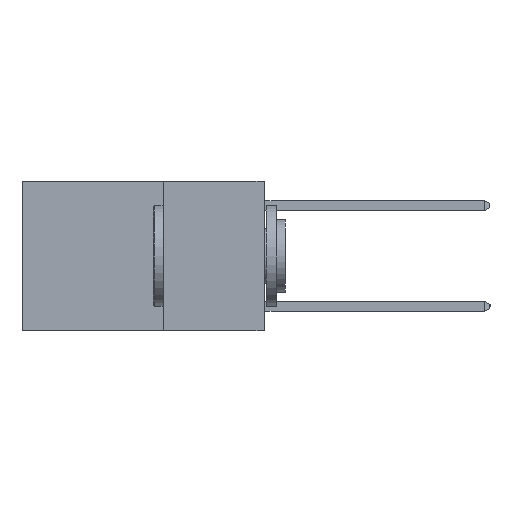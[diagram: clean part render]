
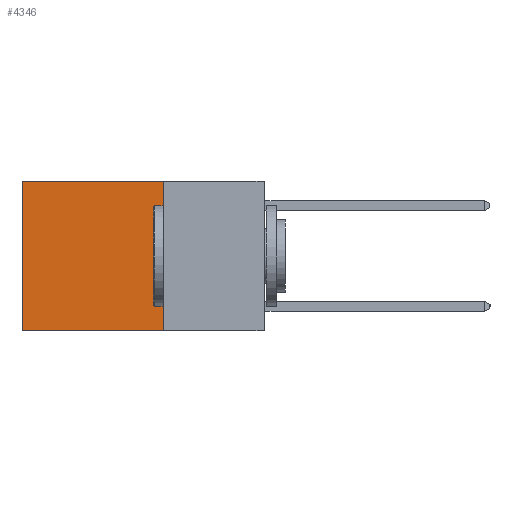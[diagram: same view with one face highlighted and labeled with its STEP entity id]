
A CAD part, left-side view. The second image highlights one B-rep face of the part: STEP entity #4346.
In plain terms, the highlighted planar face has unit normal (-1, 0, 0).
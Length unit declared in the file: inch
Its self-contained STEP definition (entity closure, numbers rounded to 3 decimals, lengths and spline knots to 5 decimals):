
#273 = LINE ( 'NONE', #6829, #2418 ) ;
#440 = EDGE_LOOP ( 'NONE', ( #10818, #9083, #8532, #10730 ) ) ;
#696 = CARTESIAN_POINT ( 'NONE',  ( 0.2625, 0.6, 0. ) ) ;
#1049 = VECTOR ( 'NONE', #3504, 39.37008 ) ;
#1800 = PLANE ( 'NONE',  #2307 ) ;
#2307 = AXIS2_PLACEMENT_3D ( 'NONE', #8114, #9018, #3644 ) ;
#2406 = VECTOR ( 'NONE', #5692, 39.37008 ) ;
#2418 = VECTOR ( 'NONE', #9549, 39.37008 ) ;
#2789 = VERTEX_POINT ( 'NONE', #3888 ) ;
#3504 = DIRECTION ( 'NONE',  ( 0., 0., -1. ) ) ;
#3644 = DIRECTION ( 'NONE',  ( 0., 0., -1. ) ) ;
#3888 = CARTESIAN_POINT ( 'NONE',  ( 0.2625, 0.25, -0.37 ) ) ;
#4155 = DIRECTION ( 'NONE',  ( 0., 0., -1. ) ) ;
#4346 = ADVANCED_FACE ( 'NONE', ( #10606 ), #1800, .F. ) ;
#4493 = VERTEX_POINT ( 'NONE', #11077 ) ;
#4801 = CARTESIAN_POINT ( 'NONE',  ( 0.2625, 0.25, -0.37 ) ) ;
#4871 = LINE ( 'NONE', #4801, #2406 ) ;
#4965 = VECTOR ( 'NONE', #4155, 39.37008 ) ;
#5692 = DIRECTION ( 'NONE',  ( 0., 1., 0. ) ) ;
#5932 = LINE ( 'NONE', #696, #1049 ) ;
#6305 = EDGE_CURVE ( 'NONE', #11323, #2789, #7295, .T. ) ;
#6829 = CARTESIAN_POINT ( 'NONE',  ( 0.2625, 0.25, 0. ) ) ;
#7295 = LINE ( 'NONE', #8602, #4965 ) ;
#8076 = EDGE_CURVE ( 'NONE', #11323, #10137, #273, .T. ) ;
#8114 = CARTESIAN_POINT ( 'NONE',  ( 0.2625, 0.25, 0. ) ) ;
#8518 = EDGE_CURVE ( 'NONE', #2789, #4493, #4871, .T. ) ;
#8532 = ORIENTED_EDGE ( 'NONE', *, *, #6305, .F. ) ;
#8602 = CARTESIAN_POINT ( 'NONE',  ( 0.2625, 0.25, 0. ) ) ;
#9018 = DIRECTION ( 'NONE',  ( 1., 0., 0. ) ) ;
#9083 = ORIENTED_EDGE ( 'NONE', *, *, #8518, .F. ) ;
#9147 = CARTESIAN_POINT ( 'NONE',  ( 0.2625, 0.25, 0. ) ) ;
#9549 = DIRECTION ( 'NONE',  ( 0., 1., 0. ) ) ;
#10137 = VERTEX_POINT ( 'NONE', #10294 ) ;
#10294 = CARTESIAN_POINT ( 'NONE',  ( 0.2625, 0.6, 0. ) ) ;
#10606 = FACE_OUTER_BOUND ( 'NONE', #440, .T. ) ;
#10730 = ORIENTED_EDGE ( 'NONE', *, *, #8076, .T. ) ;
#10818 = ORIENTED_EDGE ( 'NONE', *, *, #11033, .T. ) ;
#11033 = EDGE_CURVE ( 'NONE', #10137, #4493, #5932, .T. ) ;
#11077 = CARTESIAN_POINT ( 'NONE',  ( 0.2625, 0.6, -0.37 ) ) ;
#11323 = VERTEX_POINT ( 'NONE', #9147 ) ;
